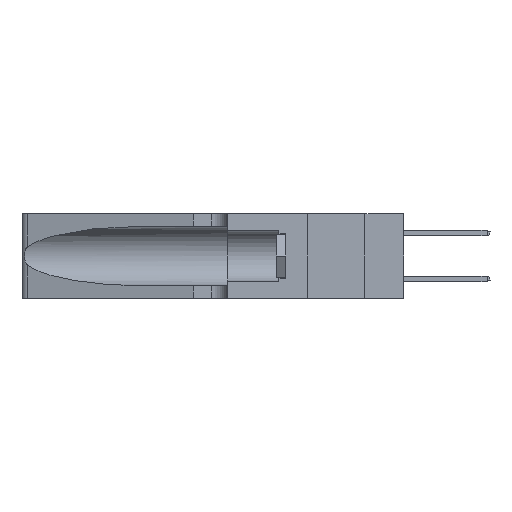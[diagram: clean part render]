
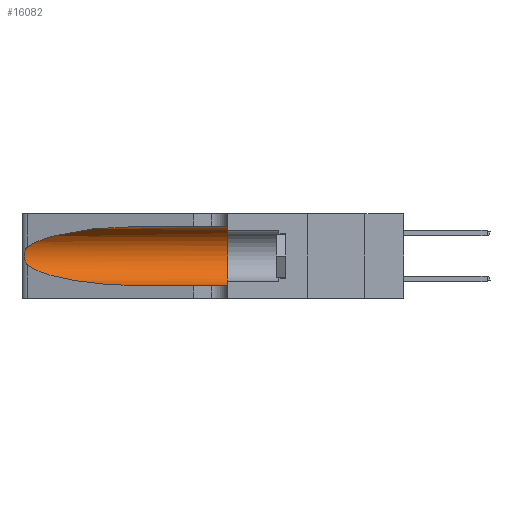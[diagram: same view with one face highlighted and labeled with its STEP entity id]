
A CAD part, left-side view. The second image highlights one B-rep face of the part: STEP entity #16082.
In plain terms, the highlighted cylindrical face has radius 3.308 mm (diameter 6.617 mm), a partial arc.
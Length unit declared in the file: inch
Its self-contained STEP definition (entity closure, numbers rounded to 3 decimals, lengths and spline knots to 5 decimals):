
#335 = VERTEX_POINT ( 'NONE', #6293 ) ;
#1087 = DIRECTION ( 'NONE',  ( 0., 0., -1. ) ) ;
#1257 = CARTESIAN_POINT ( 'NONE',  ( 0.25487, 1.22718, 0.22369 ) ) ;
#1787 = DIRECTION ( 'NONE',  ( 0., 1., 0. ) ) ;
#1793 = DIRECTION ( 'NONE',  ( 0., -1., 0. ) ) ;
#1899 = VECTOR ( 'NONE', #6477, 39.37008 ) ;
#2521 = CARTESIAN_POINT ( 'NONE',  ( 0.2373, 1.15595, 0.28018 ) ) ;
#2731 = CARTESIAN_POINT ( 'NONE',  ( 0.25639, 1.23184, 0.21858 ) ) ;
#2778 = CARTESIAN_POINT ( 'NONE',  ( 0.25487, 1.22718, 0.22369 ) ) ;
#3048 = CARTESIAN_POINT ( 'NONE',  ( 0.26017, 1.23833, 0.17102 ) ) ;
#3342 = CARTESIAN_POINT ( 'NONE',  ( 0.1305, 0.72297, 0.05475 ) ) ;
#3474 = CARTESIAN_POINT ( 'NONE',  ( 0.25487, 1.22718, 0.22369 ) ) ;
#3654 = VERTEX_POINT ( 'NONE', #22918 ) ;
#4274 = ORIENTED_EDGE ( 'NONE', *, *, #14194, .T. ) ;
#4275 = CARTESIAN_POINT ( 'NONE',  ( 0.1305, 0.72297, 0.31525 ) ) ;
#4805 = DIRECTION ( 'NONE',  ( 0., -1., 0. ) ) ;
#4851 = CYLINDRICAL_SURFACE ( 'NONE', #12216, 0.13025 ) ;
#4888 = CARTESIAN_POINT ( 'NONE',  ( 0.1305, 0.72297, 0.05475 ) ) ;
#5865 = LINE ( 'NONE', #14136, #18910 ) ;
#6293 = CARTESIAN_POINT ( 'NONE',  ( 0.25487, 1.22718, 0.14631 ) ) ;
#6477 = DIRECTION ( 'NONE',  ( 0., -1., 0. ) ) ;
#6815 = CARTESIAN_POINT ( 'NONE',  ( 0.25555, 1.22993, 0.14849 ) ) ;
#7214 = CARTESIAN_POINT ( 'NONE',  ( 0.1305, 0.35, 0.185 ) ) ;
#7798 = CARTESIAN_POINT ( 'NONE',  ( 0.18966, 0.96281, 0.31525 ) ) ;
#8170 = ORIENTED_EDGE ( 'NONE', *, *, #19481, .F. ) ;
#8308 = LINE ( 'NONE', #9716, #1899 ) ;
#8530 = CARTESIAN_POINT ( 'NONE',  ( 0.18966, 0.96281, 0.05475 ) ) ;
#8571 = CARTESIAN_POINT ( 'NONE',  ( 0.1305, 0.35, 0.05475 ) ) ;
#9004 = VERTEX_POINT ( 'NONE', #4275 ) ;
#9106 = VERTEX_POINT ( 'NONE', #3474 ) ;
#9156 =( BOUNDED_CURVE ( )  B_SPLINE_CURVE ( 3, ( #20438, #7798, #2521, #2778 ),
 .UNSPECIFIED., .F., .F. ) 
 B_SPLINE_CURVE_WITH_KNOTS ( ( 4, 4 ),
 ( 1.5708, 2.84003 ),
 .UNSPECIFIED. ) 
 CURVE ( )  GEOMETRIC_REPRESENTATION_ITEM ( )  RATIONAL_B_SPLINE_CURVE ( ( 1., 0.87, 0.87, 1. ) ) 
 REPRESENTATION_ITEM ( '' )  );
#9662 = CARTESIAN_POINT ( 'NONE',  ( 0.25854, 1.2359, 0.20912 ) ) ;
#9716 = CARTESIAN_POINT ( 'NONE',  ( 0.1305, 1.61858, 0.31525 ) ) ;
#10301 = CARTESIAN_POINT ( 'NONE',  ( 0.25789, 1.23486, 0.15765 ) ) ;
#11251 = AXIS2_PLACEMENT_3D ( 'NONE', #7214, #1787, #14418 ) ;
#11766 = CARTESIAN_POINT ( 'NONE',  ( 0.25487, 1.22718, 0.14631 ) ) ;
#11997 = CARTESIAN_POINT ( 'NONE',  ( 0.26075, 1.23896, 0.178 ) ) ;
#12216 = AXIS2_PLACEMENT_3D ( 'NONE', #14699, #4805, #1087 ) ;
#12889 = ORIENTED_EDGE ( 'NONE', *, *, #13527, .T. ) ;
#13174 = CARTESIAN_POINT ( 'NONE',  ( 0.26018, 1.23835, 0.19895 ) ) ;
#13527 = EDGE_CURVE ( 'NONE', #9004, #9106, #9156, .T. ) ;
#13790 = VERTEX_POINT ( 'NONE', #8571 ) ;
#14136 = CARTESIAN_POINT ( 'NONE',  ( 0.1305, 1.61858, 0.05475 ) ) ;
#14194 = EDGE_CURVE ( 'NONE', #9106, #335, #21932, .T. ) ;
#14418 = DIRECTION ( 'NONE',  ( 0., 0., 1. ) ) ;
#14699 = CARTESIAN_POINT ( 'NONE',  ( 0.1305, 1.61858, 0.185 ) ) ;
#15267 = CARTESIAN_POINT ( 'NONE',  ( 0.25555, 1.22994, 0.2215 ) ) ;
#15367 = EDGE_CURVE ( 'NONE', #3654, #13790, #18986, .T. ) ;
#16082 = ADVANCED_FACE ( 'NONE', ( #17348 ), #4851, .F. ) ;
#16545 = ORIENTED_EDGE ( 'NONE', *, *, #21466, .T. ) ;
#16734 = CARTESIAN_POINT ( 'NONE',  ( 0.25787, 1.23484, 0.2124 ) ) ;
#17192 = EDGE_LOOP ( 'NONE', ( #12889, #4274, #16545, #20332, #19434, #8170 ) ) ;
#17348 = FACE_OUTER_BOUND ( 'NONE', #17192, .T. ) ;
#17445 = CARTESIAN_POINT ( 'NONE',  ( 0.25856, 1.23593, 0.16098 ) ) ;
#17607 = CARTESIAN_POINT ( 'NONE',  ( 0.2373, 1.15595, 0.08982 ) ) ;
#18910 = VECTOR ( 'NONE', #1793, 39.37008 ) ;
#18986 = CIRCLE ( 'NONE', #11251, 0.13025 ) ;
#19434 = ORIENTED_EDGE ( 'NONE', *, *, #15367, .F. ) ;
#19481 = EDGE_CURVE ( 'NONE', #9004, #3654, #8308, .T. ) ;
#20245 =( BOUNDED_CURVE ( )  B_SPLINE_CURVE ( 3, ( #22703, #17607, #8530, #3342 ),
 .UNSPECIFIED., .F., .T. ) 
 B_SPLINE_CURVE_WITH_KNOTS ( ( 4, 4 ),
 ( 3.44316, 4.71239 ),
 .UNSPECIFIED. ) 
 CURVE ( )  GEOMETRIC_REPRESENTATION_ITEM ( )  RATIONAL_B_SPLINE_CURVE ( ( 1., 0.87, 0.87, 1. ) ) 
 REPRESENTATION_ITEM ( '' )  );
#20332 = ORIENTED_EDGE ( 'NONE', *, *, #20976, .T. ) ;
#20438 = CARTESIAN_POINT ( 'NONE',  ( 0.1305, 0.72297, 0.31525 ) ) ;
#20976 = EDGE_CURVE ( 'NONE', #21366, #13790, #5865, .T. ) ;
#21366 = VERTEX_POINT ( 'NONE', #4888 ) ;
#21466 = EDGE_CURVE ( 'NONE', #335, #21366, #20245, .T. ) ;
#21932 = B_SPLINE_CURVE_WITH_KNOTS ( 'NONE', 3,
 ( #1257, #15267, #2731, #16734, #9662, #13174, #22217, #11997, #3048, #17445, #10301, #22693, #6815, #11766 ),
 .UNSPECIFIED., .F., .F.,
 ( 4, 2, 2, 2, 2, 2, 4 ),
 ( 0., 0.00027, 0.00053, 0.00107, 0.0016, 0.00187, 0.00214 ),
 .UNSPECIFIED. ) ;
#22217 = CARTESIAN_POINT ( 'NONE',  ( 0.26075, 1.23896, 0.19203 ) ) ;
#22693 = CARTESIAN_POINT ( 'NONE',  ( 0.25639, 1.23186, 0.15144 ) ) ;
#22703 = CARTESIAN_POINT ( 'NONE',  ( 0.25487, 1.22718, 0.14631 ) ) ;
#22918 = CARTESIAN_POINT ( 'NONE',  ( 0.1305, 0.35, 0.31525 ) ) ;
